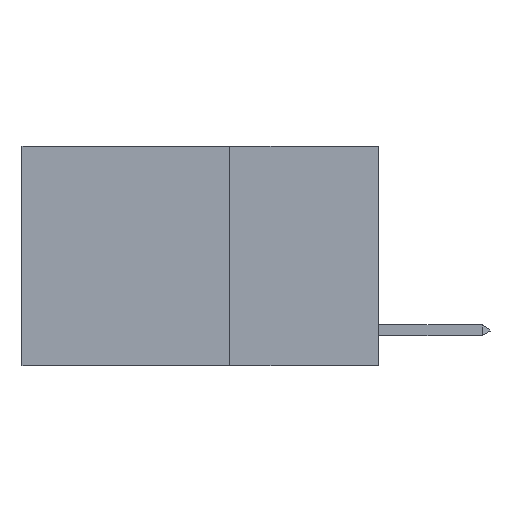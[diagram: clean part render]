
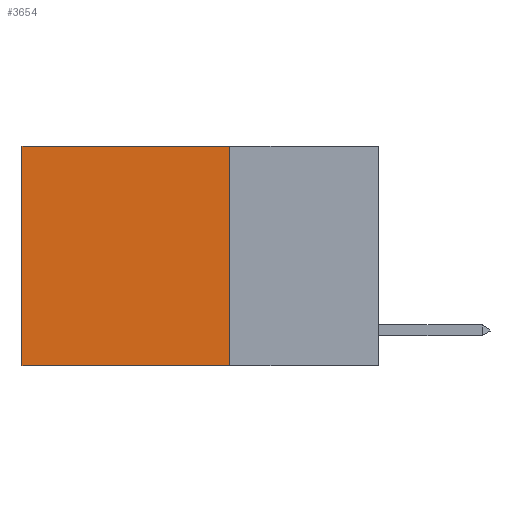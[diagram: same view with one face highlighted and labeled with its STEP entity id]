
A CAD part, left-side view. The second image highlights one B-rep face of the part: STEP entity #3654.
In plain terms, the highlighted planar face has unit normal (-1, 0, 0).
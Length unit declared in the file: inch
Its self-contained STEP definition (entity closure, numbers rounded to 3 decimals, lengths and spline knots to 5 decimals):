
#248 = DIRECTION ( 'NONE',  ( 0., 0., -1. ) ) ;
#280 = CARTESIAN_POINT ( 'NONE',  ( 0.2625, 0.6, 0. ) ) ;
#326 = VECTOR ( 'NONE', #9144, 39.37008 ) ;
#654 = VERTEX_POINT ( 'NONE', #2706 ) ;
#2018 = EDGE_LOOP ( 'NONE', ( #5823, #7544, #10547, #6901 ) ) ;
#2450 = CARTESIAN_POINT ( 'NONE',  ( 0.2625, 0.25, 0. ) ) ;
#2647 = CARTESIAN_POINT ( 'NONE',  ( 0.2625, 0.25, -0.37 ) ) ;
#2706 = CARTESIAN_POINT ( 'NONE',  ( 0.2625, 0.25, -0.37 ) ) ;
#3413 = VERTEX_POINT ( 'NONE', #11911 ) ;
#3654 = ADVANCED_FACE ( 'NONE', ( #13237 ), #11151, .F. ) ;
#3942 = DIRECTION ( 'NONE',  ( 0., 1., 0. ) ) ;
#4671 = DIRECTION ( 'NONE',  ( 0., 0., -1. ) ) ;
#4704 = EDGE_CURVE ( 'NONE', #8949, #654, #5817, .T. ) ;
#5234 = CARTESIAN_POINT ( 'NONE',  ( 0.2625, 0.25, 0. ) ) ;
#5817 = LINE ( 'NONE', #12613, #6168 ) ;
#5823 = ORIENTED_EDGE ( 'NONE', *, *, #12710, .T. ) ;
#6023 = DIRECTION ( 'NONE',  ( 0., 0., -1. ) ) ;
#6168 = VECTOR ( 'NONE', #6023, 39.37008 ) ;
#6284 = AXIS2_PLACEMENT_3D ( 'NONE', #2450, #6804, #248 ) ;
#6725 = VECTOR ( 'NONE', #4671, 39.37008 ) ;
#6804 = DIRECTION ( 'NONE',  ( 1., 0., 0. ) ) ;
#6901 = ORIENTED_EDGE ( 'NONE', *, *, #13445, .T. ) ;
#7544 = ORIENTED_EDGE ( 'NONE', *, *, #10488, .F. ) ;
#8949 = VERTEX_POINT ( 'NONE', #5234 ) ;
#9035 = LINE ( 'NONE', #2647, #326 ) ;
#9144 = DIRECTION ( 'NONE',  ( 0., 1., 0. ) ) ;
#9254 = LINE ( 'NONE', #13814, #12567 ) ;
#9611 = LINE ( 'NONE', #280, #6725 ) ;
#10488 = EDGE_CURVE ( 'NONE', #654, #3413, #9035, .T. ) ;
#10547 = ORIENTED_EDGE ( 'NONE', *, *, #4704, .F. ) ;
#10592 = CARTESIAN_POINT ( 'NONE',  ( 0.2625, 0.6, 0. ) ) ;
#11151 = PLANE ( 'NONE',  #6284 ) ;
#11911 = CARTESIAN_POINT ( 'NONE',  ( 0.2625, 0.6, -0.37 ) ) ;
#12386 = VERTEX_POINT ( 'NONE', #10592 ) ;
#12567 = VECTOR ( 'NONE', #3942, 39.37008 ) ;
#12613 = CARTESIAN_POINT ( 'NONE',  ( 0.2625, 0.25, 0. ) ) ;
#12710 = EDGE_CURVE ( 'NONE', #12386, #3413, #9611, .T. ) ;
#13237 = FACE_OUTER_BOUND ( 'NONE', #2018, .T. ) ;
#13445 = EDGE_CURVE ( 'NONE', #8949, #12386, #9254, .T. ) ;
#13814 = CARTESIAN_POINT ( 'NONE',  ( 0.2625, 0.25, 0. ) ) ;
